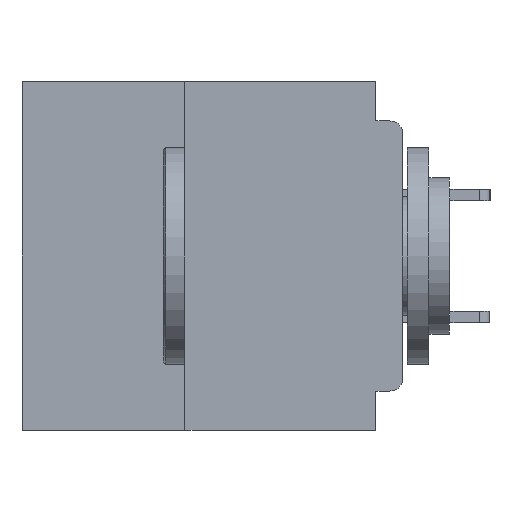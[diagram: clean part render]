
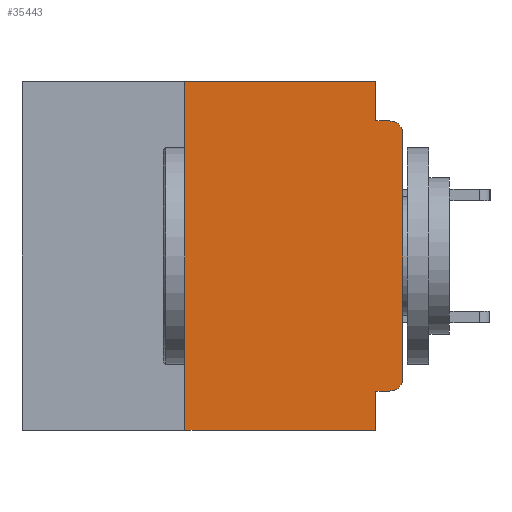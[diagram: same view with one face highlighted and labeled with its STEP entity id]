
A CAD part, left-side view. The second image highlights one B-rep face of the part: STEP entity #35443.
In plain terms, the highlighted planar face has unit normal (-1, 0, 0).
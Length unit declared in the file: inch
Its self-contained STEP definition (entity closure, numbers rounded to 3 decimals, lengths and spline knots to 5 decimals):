
#246 = ORIENTED_EDGE ( 'NONE', *, *, #65698, .T. ) ;
#296 = VECTOR ( 'NONE', #62192, 39.37008 ) ;
#2272 = CARTESIAN_POINT ( 'NONE',  ( 0., 0.015, -0.355 ) ) ;
#3372 = CARTESIAN_POINT ( 'NONE',  ( 0., 0.015, -0.045 ) ) ;
#5052 = VERTEX_POINT ( 'NONE', #56605 ) ;
#5479 = EDGE_CURVE ( 'NONE', #59833, #64490, #15095, .T. ) ;
#6020 = CIRCLE ( 'NONE', #26835, 0.015 ) ;
#6328 = CARTESIAN_POINT ( 'NONE',  ( 0., 0.031, -0.4 ) ) ;
#8077 = LINE ( 'NONE', #14905, #20246 ) ;
#10356 = DIRECTION ( 'NONE',  ( -1., 0., 0. ) ) ;
#11015 = LINE ( 'NONE', #56565, #62715 ) ;
#11500 = VECTOR ( 'NONE', #27415, 39.37008 ) ;
#11598 = EDGE_CURVE ( 'NONE', #59833, #5052, #30506, .T. ) ;
#12338 = EDGE_CURVE ( 'NONE', #19796, #62160, #20637, .T. ) ;
#13517 = CARTESIAN_POINT ( 'NONE',  ( 0., 0.437, 0. ) ) ;
#14905 = CARTESIAN_POINT ( 'NONE',  ( 0., 0.031, -0.4 ) ) ;
#15095 = LINE ( 'NONE', #23862, #54714 ) ;
#15376 = EDGE_LOOP ( 'NONE', ( #246, #48914, #58512, #24049, #31161, #66212, #54025, #38976, #28725, #42631 ) ) ;
#15437 = EDGE_CURVE ( 'NONE', #26540, #17183, #6020, .T. ) ;
#15965 = CARTESIAN_POINT ( 'NONE',  ( 0., 0.437, -0.4 ) ) ;
#17045 = DIRECTION ( 'NONE',  ( 0., 0., 1. ) ) ;
#17183 = VERTEX_POINT ( 'NONE', #3372 ) ;
#18889 = EDGE_CURVE ( 'NONE', #62214, #58119, #53293, .T. ) ;
#19173 = CARTESIAN_POINT ( 'NONE',  ( 0., 0.031, -0.355 ) ) ;
#19796 = VERTEX_POINT ( 'NONE', #65072 ) ;
#20246 = VECTOR ( 'NONE', #66554, 39.37008 ) ;
#20289 = DIRECTION ( 'NONE',  ( -1., 0., 0. ) ) ;
#20465 = DIRECTION ( 'NONE',  ( 0., 0., 1. ) ) ;
#20637 = LINE ( 'NONE', #15965, #296 ) ;
#23319 = PLANE ( 'NONE',  #32898 ) ;
#23862 = CARTESIAN_POINT ( 'NONE',  ( 0., 0., -0.355 ) ) ;
#24049 = ORIENTED_EDGE ( 'NONE', *, *, #18889, .F. ) ;
#24821 = VECTOR ( 'NONE', #49890, 39.37008 ) ;
#26540 = VERTEX_POINT ( 'NONE', #47122 ) ;
#26835 = AXIS2_PLACEMENT_3D ( 'NONE', #51213, #20289, #56387 ) ;
#27198 = CARTESIAN_POINT ( 'NONE',  ( 0., 0.031, 0. ) ) ;
#27415 = DIRECTION ( 'NONE',  ( 0., -1., 0. ) ) ;
#28725 = ORIENTED_EDGE ( 'NONE', *, *, #5479, .F. ) ;
#29122 = DIRECTION ( 'NONE',  ( 0., 1., 0. ) ) ;
#30506 = CIRCLE ( 'NONE', #42603, 0.015 ) ;
#31161 = ORIENTED_EDGE ( 'NONE', *, *, #39890, .F. ) ;
#32898 = AXIS2_PLACEMENT_3D ( 'NONE', #59395, #64546, #33792 ) ;
#33792 = DIRECTION ( 'NONE',  ( 0., 0., -1. ) ) ;
#35443 = ADVANCED_FACE ( 'NONE', ( #38556 ), #23319, .F. ) ;
#37977 = VECTOR ( 'NONE', #52878, 39.37008 ) ;
#38556 = FACE_OUTER_BOUND ( 'NONE', #15376, .T. ) ;
#38599 = LINE ( 'NONE', #13517, #24821 ) ;
#38976 = ORIENTED_EDGE ( 'NONE', *, *, #60654, .F. ) ;
#39890 = EDGE_CURVE ( 'NONE', #56268, #62214, #38599, .T. ) ;
#40352 = LINE ( 'NONE', #63267, #50755 ) ;
#41414 = CARTESIAN_POINT ( 'NONE',  ( 0., 0.015, -0.34 ) ) ;
#42603 = AXIS2_PLACEMENT_3D ( 'NONE', #41414, #10356, #46545 ) ;
#42631 = ORIENTED_EDGE ( 'NONE', *, *, #11598, .T. ) ;
#42963 = CARTESIAN_POINT ( 'NONE',  ( 0., 0., -0.045 ) ) ;
#46433 = CARTESIAN_POINT ( 'NONE',  ( 0., 0.25, 0. ) ) ;
#46545 = DIRECTION ( 'NONE',  ( 0., 0., -1. ) ) ;
#47122 = CARTESIAN_POINT ( 'NONE',  ( 0., 0., -0.06 ) ) ;
#48914 = ORIENTED_EDGE ( 'NONE', *, *, #15437, .T. ) ;
#49890 = DIRECTION ( 'NONE',  ( 0., -1., 0. ) ) ;
#50755 = VECTOR ( 'NONE', #17045, 39.37008 ) ;
#51134 = LINE ( 'NONE', #42963, #11500 ) ;
#51213 = CARTESIAN_POINT ( 'NONE',  ( 0., 0.015, -0.06 ) ) ;
#52878 = DIRECTION ( 'NONE',  ( 0., 0., -1. ) ) ;
#53293 = LINE ( 'NONE', #27198, #37977 ) ;
#53972 = CARTESIAN_POINT ( 'NONE',  ( 0., 0.031, -0.045 ) ) ;
#54025 = ORIENTED_EDGE ( 'NONE', *, *, #12338, .T. ) ;
#54714 = VECTOR ( 'NONE', #29122, 39.37008 ) ;
#56228 = EDGE_CURVE ( 'NONE', #19796, #56268, #11015, .T. ) ;
#56268 = VERTEX_POINT ( 'NONE', #46433 ) ;
#56387 = DIRECTION ( 'NONE',  ( 0., 0., -1. ) ) ;
#56565 = CARTESIAN_POINT ( 'NONE',  ( 0., 0.25, -0.4 ) ) ;
#56605 = CARTESIAN_POINT ( 'NONE',  ( 0., 0., -0.34 ) ) ;
#58119 = VERTEX_POINT ( 'NONE', #53972 ) ;
#58308 = CARTESIAN_POINT ( 'NONE',  ( 0., 0.031, 0. ) ) ;
#58512 = ORIENTED_EDGE ( 'NONE', *, *, #62504, .F. ) ;
#59395 = CARTESIAN_POINT ( 'NONE',  ( 0., 0.437, 0. ) ) ;
#59833 = VERTEX_POINT ( 'NONE', #2272 ) ;
#60654 = EDGE_CURVE ( 'NONE', #64490, #62160, #8077, .T. ) ;
#62160 = VERTEX_POINT ( 'NONE', #6328 ) ;
#62192 = DIRECTION ( 'NONE',  ( 0., -1., 0. ) ) ;
#62214 = VERTEX_POINT ( 'NONE', #58308 ) ;
#62504 = EDGE_CURVE ( 'NONE', #58119, #17183, #51134, .T. ) ;
#62715 = VECTOR ( 'NONE', #20465, 39.37008 ) ;
#63267 = CARTESIAN_POINT ( 'NONE',  ( 0., 0., 0. ) ) ;
#64490 = VERTEX_POINT ( 'NONE', #19173 ) ;
#64546 = DIRECTION ( 'NONE',  ( 1., 0., 0. ) ) ;
#65072 = CARTESIAN_POINT ( 'NONE',  ( 0., 0.25, -0.4 ) ) ;
#65698 = EDGE_CURVE ( 'NONE', #5052, #26540, #40352, .T. ) ;
#66212 = ORIENTED_EDGE ( 'NONE', *, *, #56228, .F. ) ;
#66554 = DIRECTION ( 'NONE',  ( 0., 0., -1. ) ) ;
